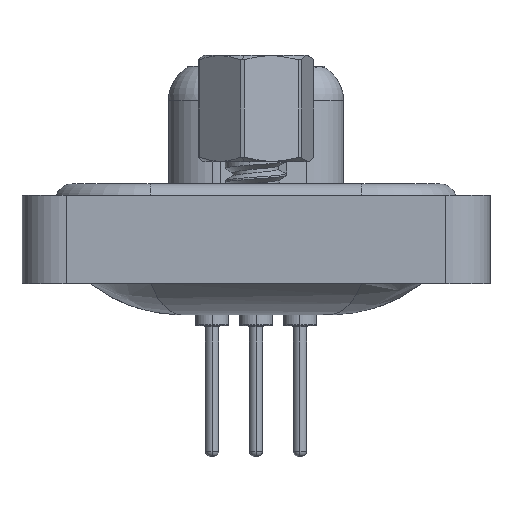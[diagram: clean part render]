
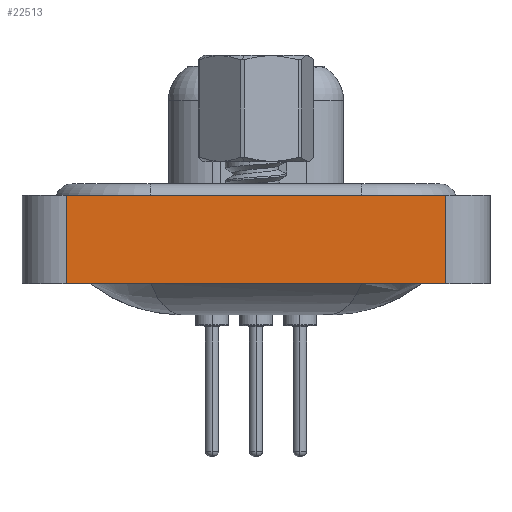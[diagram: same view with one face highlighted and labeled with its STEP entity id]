
A CAD part, left-side view. The second image highlights one B-rep face of the part: STEP entity #22513.
In plain terms, the highlighted planar face has unit normal (-1, 0, 0).
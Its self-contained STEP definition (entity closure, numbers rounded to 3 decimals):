
#346 = CARTESIAN_POINT ( 'NONE',  ( -7.26, 8.55, -3.6 ) ) ;
#943 = CARTESIAN_POINT ( 'NONE',  ( -7.26, -8.55, -3.6 ) ) ;
#1100 = VECTOR ( 'NONE', #7765, 1000. ) ;
#1321 = ORIENTED_EDGE ( 'NONE', *, *, #6408, .F. ) ;
#1513 = LINE ( 'NONE', #7439, #21634 ) ;
#3778 = LINE ( 'NONE', #15993, #1100 ) ;
#4828 = CARTESIAN_POINT ( 'NONE',  ( -7.26, -8.55, -3.6 ) ) ;
#5369 = EDGE_CURVE ( 'NONE', #20690, #24480, #3778, .T. ) ;
#5505 = VERTEX_POINT ( 'NONE', #8662 ) ;
#6408 = EDGE_CURVE ( 'NONE', #20690, #5505, #17972, .T. ) ;
#6998 = DIRECTION ( 'NONE',  ( 0., 0., 1. ) ) ;
#7363 = VERTEX_POINT ( 'NONE', #13929 ) ;
#7371 = VECTOR ( 'NONE', #8833, 1000. ) ;
#7439 = CARTESIAN_POINT ( 'NONE',  ( -7.26, -8.55, 0.4 ) ) ;
#7765 = DIRECTION ( 'NONE',  ( 0., -1., 0. ) ) ;
#8364 = EDGE_LOOP ( 'NONE', ( #11132, #13995, #1321, #15365 ) ) ;
#8662 = CARTESIAN_POINT ( 'NONE',  ( -7.26, 8.55, 0.4 ) ) ;
#8833 = DIRECTION ( 'NONE',  ( 0., 0., 1. ) ) ;
#9438 = LINE ( 'NONE', #9809, #14667 ) ;
#9809 = CARTESIAN_POINT ( 'NONE',  ( -7.26, -8.55, -3.6 ) ) ;
#11132 = ORIENTED_EDGE ( 'NONE', *, *, #22707, .T. ) ;
#11549 = DIRECTION ( 'NONE',  ( 0., -1., 0. ) ) ;
#12919 = PLANE ( 'NONE',  #14685 ) ;
#13929 = CARTESIAN_POINT ( 'NONE',  ( -7.26, -8.55, 0.4 ) ) ;
#13995 = ORIENTED_EDGE ( 'NONE', *, *, #23598, .F. ) ;
#14667 = VECTOR ( 'NONE', #17647, 1000. ) ;
#14685 = AXIS2_PLACEMENT_3D ( 'NONE', #943, #18840, #6998 ) ;
#15365 = ORIENTED_EDGE ( 'NONE', *, *, #5369, .T. ) ;
#15993 = CARTESIAN_POINT ( 'NONE',  ( -7.26, -8.55, -3.6 ) ) ;
#17647 = DIRECTION ( 'NONE',  ( 0., 0., 1. ) ) ;
#17972 = LINE ( 'NONE', #346, #7371 ) ;
#18840 = DIRECTION ( 'NONE',  ( -1., 0., 0. ) ) ;
#19235 = CARTESIAN_POINT ( 'NONE',  ( -7.26, 8.55, -3.6 ) ) ;
#20690 = VERTEX_POINT ( 'NONE', #19235 ) ;
#20893 = FACE_OUTER_BOUND ( 'NONE', #8364, .T. ) ;
#21634 = VECTOR ( 'NONE', #11549, 1000. ) ;
#22513 = ADVANCED_FACE ( 'NONE', ( #20893 ), #12919, .T. ) ;
#22707 = EDGE_CURVE ( 'NONE', #24480, #7363, #9438, .T. ) ;
#23598 = EDGE_CURVE ( 'NONE', #5505, #7363, #1513, .T. ) ;
#24480 = VERTEX_POINT ( 'NONE', #4828 ) ;
